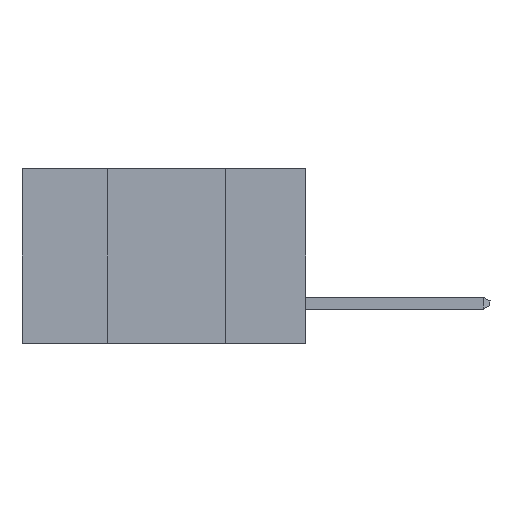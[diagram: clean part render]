
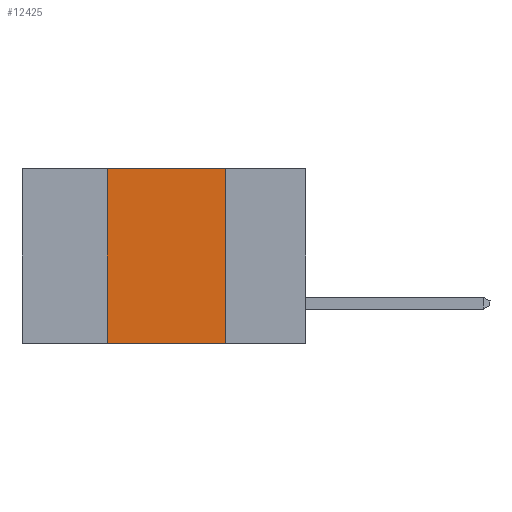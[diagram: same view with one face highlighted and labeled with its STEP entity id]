
A CAD part, left-side view. The second image highlights one B-rep face of the part: STEP entity #12425.
In plain terms, the highlighted planar face has unit normal (-1, 0, 0).
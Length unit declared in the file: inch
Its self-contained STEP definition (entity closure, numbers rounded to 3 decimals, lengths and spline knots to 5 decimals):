
#7 = CARTESIAN_POINT ( 'NONE',  ( 0., 0.17, 0. ) ) ;
#162 = VERTEX_POINT ( 'NONE', #20036 ) ;
#311 = VECTOR ( 'NONE', #16484, 39.37008 ) ;
#963 = DIRECTION ( 'NONE',  ( 1., 0., 0. ) ) ;
#1469 = CARTESIAN_POINT ( 'NONE',  ( 0., 0.17, -0.37 ) ) ;
#2997 = VECTOR ( 'NONE', #14184, 39.37008 ) ;
#3454 = EDGE_CURVE ( 'NONE', #162, #13428, #6555, .T. ) ;
#4123 = ORIENTED_EDGE ( 'NONE', *, *, #8506, .F. ) ;
#4637 = CARTESIAN_POINT ( 'NONE',  ( 0., 0.42, 0. ) ) ;
#5441 = AXIS2_PLACEMENT_3D ( 'NONE', #6096, #963, #16894 ) ;
#6096 = CARTESIAN_POINT ( 'NONE',  ( 0., 0.6, 0. ) ) ;
#6555 = LINE ( 'NONE', #11667, #9252 ) ;
#6869 = CARTESIAN_POINT ( 'NONE',  ( 0., 0.6, 0. ) ) ;
#6973 = VERTEX_POINT ( 'NONE', #7 ) ;
#7405 = CARTESIAN_POINT ( 'NONE',  ( 0., 0.17, -0.37 ) ) ;
#8506 = EDGE_CURVE ( 'NONE', #6973, #13428, #8932, .T. ) ;
#8932 = LINE ( 'NONE', #7405, #311 ) ;
#9252 = VECTOR ( 'NONE', #19007, 39.37008 ) ;
#9836 = ORIENTED_EDGE ( 'NONE', *, *, #15087, .F. ) ;
#10035 = VERTEX_POINT ( 'NONE', #4637 ) ;
#11667 = CARTESIAN_POINT ( 'NONE',  ( 0., 0.6, -0.37 ) ) ;
#12425 = ADVANCED_FACE ( 'NONE', ( #13518 ), #18872, .F. ) ;
#13428 = VERTEX_POINT ( 'NONE', #1469 ) ;
#13518 = FACE_OUTER_BOUND ( 'NONE', #15765, .T. ) ;
#14108 = DIRECTION ( 'NONE',  ( 0., 0., 1. ) ) ;
#14184 = DIRECTION ( 'NONE',  ( 0., -1., 0. ) ) ;
#15087 = EDGE_CURVE ( 'NONE', #162, #10035, #17493, .T. ) ;
#15765 = EDGE_LOOP ( 'NONE', ( #4123, #19057, #9836, #20820 ) ) ;
#15825 = LINE ( 'NONE', #6869, #2997 ) ;
#16484 = DIRECTION ( 'NONE',  ( 0., 0., -1. ) ) ;
#16894 = DIRECTION ( 'NONE',  ( 0., 0., -1. ) ) ;
#17493 = LINE ( 'NONE', #19586, #18154 ) ;
#18154 = VECTOR ( 'NONE', #14108, 39.37008 ) ;
#18822 = EDGE_CURVE ( 'NONE', #10035, #6973, #15825, .T. ) ;
#18872 = PLANE ( 'NONE',  #5441 ) ;
#19007 = DIRECTION ( 'NONE',  ( 0., -1., 0. ) ) ;
#19057 = ORIENTED_EDGE ( 'NONE', *, *, #18822, .F. ) ;
#19586 = CARTESIAN_POINT ( 'NONE',  ( 0., 0.42, -0.37 ) ) ;
#20036 = CARTESIAN_POINT ( 'NONE',  ( 0., 0.42, -0.37 ) ) ;
#20820 = ORIENTED_EDGE ( 'NONE', *, *, #3454, .T. ) ;
